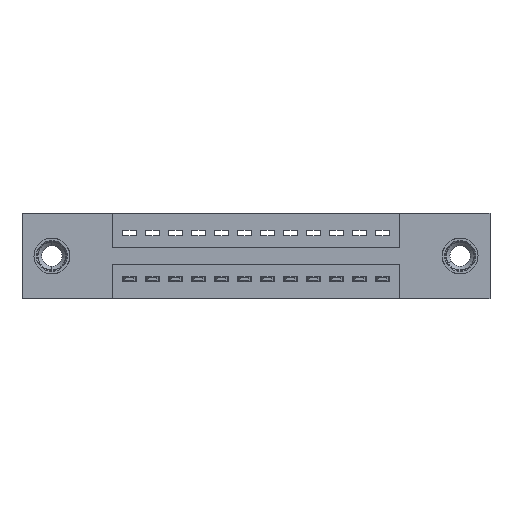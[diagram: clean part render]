
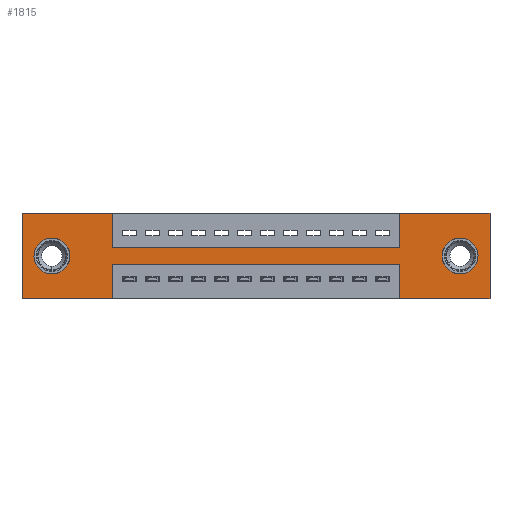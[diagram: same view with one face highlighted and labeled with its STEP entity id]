
A CAD part, front view. The second image highlights one B-rep face of the part: STEP entity #1815.
In plain terms, the highlighted planar face has unit normal (0, -1, 0).
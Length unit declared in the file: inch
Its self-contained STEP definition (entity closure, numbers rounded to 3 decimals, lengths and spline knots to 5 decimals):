
#14 = AXIS2_PLACEMENT_3D ( 'NONE', #9229, #7134, #472 ) ;
#186 = FACE_OUTER_BOUND ( 'NONE', #11313, .T. ) ;
#368 = AXIS2_PLACEMENT_3D ( 'NONE', #5534, #12993, #6627 ) ;
#423 = ORIENTED_EDGE ( 'NONE', *, *, #9155, .T. ) ;
#431 = DIRECTION ( 'NONE',  ( 0., 1., 0. ) ) ;
#470 = ORIENTED_EDGE ( 'NONE', *, *, #10024, .T. ) ;
#472 = DIRECTION ( 'NONE',  ( 0., 0., -1. ) ) ;
#623 = CARTESIAN_POINT ( 'NONE',  ( 0.3925, 0., 0. ) ) ;
#678 = CARTESIAN_POINT ( 'NONE',  ( 0.3925, 0., -0.15 ) ) ;
#856 = ORIENTED_EDGE ( 'NONE', *, *, #12166, .F. ) ;
#909 = ORIENTED_EDGE ( 'NONE', *, *, #5625, .F. ) ;
#920 = LINE ( 'NONE', #3247, #6455 ) ;
#1122 = VERTEX_POINT ( 'NONE', #12461 ) ;
#1358 = LINE ( 'NONE', #4482, #10050 ) ;
#1428 = ORIENTED_EDGE ( 'NONE', *, *, #10841, .T. ) ;
#1479 = AXIS2_PLACEMENT_3D ( 'NONE', #9365, #2869, #10458 ) ;
#1757 = VECTOR ( 'NONE', #2657, 39.37008 ) ;
#1815 = ADVANCED_FACE ( 'NONE', ( #8999, #8634, #186 ), #13470, .T. ) ;
#1885 = ORIENTED_EDGE ( 'NONE', *, *, #8242, .F. ) ;
#1908 = EDGE_CURVE ( 'NONE', #1122, #1940, #12963, .T. ) ;
#1936 = LINE ( 'NONE', #11956, #13068 ) ;
#1940 = VERTEX_POINT ( 'NONE', #678 ) ;
#2052 = CARTESIAN_POINT ( 'NONE',  ( 0., 0., -0.37 ) ) ;
#2524 = CARTESIAN_POINT ( 'NONE',  ( 1.905, 0., -0.107 ) ) ;
#2657 = DIRECTION ( 'NONE',  ( 1., 0., 0. ) ) ;
#2869 = DIRECTION ( 'NONE',  ( 0., 1., 0. ) ) ;
#3052 = CARTESIAN_POINT ( 'NONE',  ( 1.6425, 0., 0. ) ) ;
#3069 = VECTOR ( 'NONE', #8802, 39.37008 ) ;
#3229 = CIRCLE ( 'NONE', #7537, 0.078 ) ;
#3247 = CARTESIAN_POINT ( 'NONE',  ( 0., 0., 0. ) ) ;
#3285 = ORIENTED_EDGE ( 'NONE', *, *, #12752, .F. ) ;
#3389 = CARTESIAN_POINT ( 'NONE',  ( 0.3925, 0., -0.37 ) ) ;
#3502 = CARTESIAN_POINT ( 'NONE',  ( 0.13, 0., -0.185 ) ) ;
#3689 = VERTEX_POINT ( 'NONE', #13556 ) ;
#4308 = VERTEX_POINT ( 'NONE', #7169 ) ;
#4394 = CARTESIAN_POINT ( 'NONE',  ( 0.3925, 0., -0.37 ) ) ;
#4482 = CARTESIAN_POINT ( 'NONE',  ( 0., 0., 0. ) ) ;
#4618 = DIRECTION ( 'NONE',  ( 0., 0., 1. ) ) ;
#4690 = LINE ( 'NONE', #9160, #1757 ) ;
#4744 = CARTESIAN_POINT ( 'NONE',  ( 1.6425, 0., -0.22 ) ) ;
#4942 = CARTESIAN_POINT ( 'NONE',  ( 1.6425, 0., -0.37 ) ) ;
#5047 = CARTESIAN_POINT ( 'NONE',  ( 0., 0., -0.37 ) ) ;
#5121 = CARTESIAN_POINT ( 'NONE',  ( 1.6425, 0., -0.15 ) ) ;
#5132 = VERTEX_POINT ( 'NONE', #5121 ) ;
#5224 = VECTOR ( 'NONE', #12191, 39.37008 ) ;
#5233 = CARTESIAN_POINT ( 'NONE',  ( 1.905, 0., -0.263 ) ) ;
#5349 = CIRCLE ( 'NONE', #1479, 0.078 ) ;
#5367 = VERTEX_POINT ( 'NONE', #4394 ) ;
#5524 = DIRECTION ( 'NONE',  ( 1., 0., 0. ) ) ;
#5534 = CARTESIAN_POINT ( 'NONE',  ( 0.13, 0., -0.185 ) ) ;
#5580 = VERTEX_POINT ( 'NONE', #2524 ) ;
#5625 = EDGE_CURVE ( 'NONE', #13855, #11706, #11617, .T. ) ;
#6088 = EDGE_CURVE ( 'NONE', #12155, #4308, #7764, .T. ) ;
#6093 = EDGE_CURVE ( 'NONE', #6257, #1122, #1936, .T. ) ;
#6168 = ORIENTED_EDGE ( 'NONE', *, *, #13460, .F. ) ;
#6257 = VERTEX_POINT ( 'NONE', #11175 ) ;
#6318 = EDGE_CURVE ( 'NONE', #1940, #5132, #4690, .T. ) ;
#6455 = VECTOR ( 'NONE', #5524, 39.37008 ) ;
#6519 = LINE ( 'NONE', #5047, #12213 ) ;
#6586 = VERTEX_POINT ( 'NONE', #3052 ) ;
#6627 = DIRECTION ( 'NONE',  ( 0., 0., 1. ) ) ;
#6693 = LINE ( 'NONE', #2052, #9542 ) ;
#6786 = EDGE_CURVE ( 'NONE', #9084, #7261, #7770, .T. ) ;
#6898 = CARTESIAN_POINT ( 'NONE',  ( 2.035, 0., 0. ) ) ;
#7001 = LINE ( 'NONE', #4942, #11998 ) ;
#7092 = CARTESIAN_POINT ( 'NONE',  ( 1.905, 0., -0.185 ) ) ;
#7134 = DIRECTION ( 'NONE',  ( 0., -1., 0. ) ) ;
#7158 = DIRECTION ( 'NONE',  ( 0., 0., 1. ) ) ;
#7169 = CARTESIAN_POINT ( 'NONE',  ( 0.13, 0., -0.107 ) ) ;
#7261 = VERTEX_POINT ( 'NONE', #11735 ) ;
#7448 = CARTESIAN_POINT ( 'NONE',  ( 1.6425, 0., 0. ) ) ;
#7537 = AXIS2_PLACEMENT_3D ( 'NONE', #7092, #431, #8154 ) ;
#7718 = DIRECTION ( 'NONE',  ( 1., 0., 0. ) ) ;
#7721 = ORIENTED_EDGE ( 'NONE', *, *, #1908, .F. ) ;
#7764 = CIRCLE ( 'NONE', #368, 0.078 ) ;
#7770 = LINE ( 'NONE', #7787, #10628 ) ;
#7787 = CARTESIAN_POINT ( 'NONE',  ( 0.3925, 0., -0.22 ) ) ;
#7790 = ORIENTED_EDGE ( 'NONE', *, *, #6318, .F. ) ;
#8154 = DIRECTION ( 'NONE',  ( 0., 0., -1. ) ) ;
#8242 = EDGE_CURVE ( 'NONE', #3689, #6257, #1358, .T. ) ;
#8494 = DIRECTION ( 'NONE',  ( 0., 0., 1. ) ) ;
#8506 = CARTESIAN_POINT ( 'NONE',  ( 1.6425, 0., -0.37 ) ) ;
#8634 = FACE_BOUND ( 'NONE', #10811, .T. ) ;
#8802 = DIRECTION ( 'NONE',  ( 0., 0., -1. ) ) ;
#8856 = LINE ( 'NONE', #3389, #3069 ) ;
#8874 = CARTESIAN_POINT ( 'NONE',  ( 2.035, 0., -0.37 ) ) ;
#8884 = AXIS2_PLACEMENT_3D ( 'NONE', #3502, #11093, #4618 ) ;
#8886 = ORIENTED_EDGE ( 'NONE', *, *, #8948, .F. ) ;
#8948 = EDGE_CURVE ( 'NONE', #7261, #5367, #8856, .T. ) ;
#8999 = FACE_BOUND ( 'NONE', #11245, .T. ) ;
#9084 = VERTEX_POINT ( 'NONE', #4744 ) ;
#9155 = EDGE_CURVE ( 'NONE', #12105, #5580, #3229, .T. ) ;
#9160 = CARTESIAN_POINT ( 'NONE',  ( 0.3925, 0., -0.15 ) ) ;
#9229 = CARTESIAN_POINT ( 'NONE',  ( 0., 0., -0.37 ) ) ;
#9365 = CARTESIAN_POINT ( 'NONE',  ( 1.905, 0., -0.185 ) ) ;
#9406 = DIRECTION ( 'NONE',  ( 0., 0., -1. ) ) ;
#9542 = VECTOR ( 'NONE', #9651, 39.37008 ) ;
#9651 = DIRECTION ( 'NONE',  ( -1., 0., 0. ) ) ;
#10024 = EDGE_CURVE ( 'NONE', #4308, #12155, #11508, .T. ) ;
#10050 = VECTOR ( 'NONE', #11997, 39.37008 ) ;
#10148 = CARTESIAN_POINT ( 'NONE',  ( 2.035, 0., 0. ) ) ;
#10160 = VECTOR ( 'NONE', #9406, 39.37008 ) ;
#10179 = ORIENTED_EDGE ( 'NONE', *, *, #13659, .F. ) ;
#10292 = ORIENTED_EDGE ( 'NONE', *, *, #6786, .F. ) ;
#10354 = VERTEX_POINT ( 'NONE', #8506 ) ;
#10374 = VECTOR ( 'NONE', #8494, 39.37008 ) ;
#10423 = ORIENTED_EDGE ( 'NONE', *, *, #11986, .F. ) ;
#10428 = DIRECTION ( 'NONE',  ( -1., 0., 0. ) ) ;
#10458 = DIRECTION ( 'NONE',  ( 0., 0., -1. ) ) ;
#10628 = VECTOR ( 'NONE', #13071, 39.37008 ) ;
#10811 = EDGE_LOOP ( 'NONE', ( #470, #13287 ) ) ;
#10841 = EDGE_CURVE ( 'NONE', #5580, #12105, #5349, .T. ) ;
#11093 = DIRECTION ( 'NONE',  ( 0., 1., 0. ) ) ;
#11175 = CARTESIAN_POINT ( 'NONE',  ( 0., 0., 0. ) ) ;
#11245 = EDGE_LOOP ( 'NONE', ( #1428, #423 ) ) ;
#11293 = ORIENTED_EDGE ( 'NONE', *, *, #6093, .F. ) ;
#11313 = EDGE_LOOP ( 'NONE', ( #8886, #10292, #6168, #856, #909, #10179, #3285, #7790, #7721, #11293, #1885, #10423 ) ) ;
#11508 = CIRCLE ( 'NONE', #8884, 0.078 ) ;
#11617 = LINE ( 'NONE', #10148, #5224 ) ;
#11706 = VERTEX_POINT ( 'NONE', #8874 ) ;
#11715 = CARTESIAN_POINT ( 'NONE',  ( 0.13, 0., -0.263 ) ) ;
#11735 = CARTESIAN_POINT ( 'NONE',  ( 0.3925, 0., -0.22 ) ) ;
#11956 = CARTESIAN_POINT ( 'NONE',  ( 0., 0., 0. ) ) ;
#11986 = EDGE_CURVE ( 'NONE', #5367, #3689, #6519, .T. ) ;
#11997 = DIRECTION ( 'NONE',  ( 0., 0., 1. ) ) ;
#11998 = VECTOR ( 'NONE', #7158, 39.37008 ) ;
#12105 = VERTEX_POINT ( 'NONE', #5233 ) ;
#12155 = VERTEX_POINT ( 'NONE', #11715 ) ;
#12166 = EDGE_CURVE ( 'NONE', #11706, #10354, #6693, .T. ) ;
#12191 = DIRECTION ( 'NONE',  ( 0., 0., -1. ) ) ;
#12213 = VECTOR ( 'NONE', #10428, 39.37008 ) ;
#12461 = CARTESIAN_POINT ( 'NONE',  ( 0.3925, 0., 0. ) ) ;
#12752 = EDGE_CURVE ( 'NONE', #5132, #6586, #12823, .T. ) ;
#12823 = LINE ( 'NONE', #7448, #10374 ) ;
#12963 = LINE ( 'NONE', #623, #10160 ) ;
#12993 = DIRECTION ( 'NONE',  ( 0., 1., 0. ) ) ;
#13068 = VECTOR ( 'NONE', #7718, 39.37008 ) ;
#13071 = DIRECTION ( 'NONE',  ( -1., 0., 0. ) ) ;
#13287 = ORIENTED_EDGE ( 'NONE', *, *, #6088, .T. ) ;
#13460 = EDGE_CURVE ( 'NONE', #10354, #9084, #7001, .T. ) ;
#13470 = PLANE ( 'NONE',  #14 ) ;
#13556 = CARTESIAN_POINT ( 'NONE',  ( 0., 0., -0.37 ) ) ;
#13659 = EDGE_CURVE ( 'NONE', #6586, #13855, #920, .T. ) ;
#13855 = VERTEX_POINT ( 'NONE', #6898 ) ;
